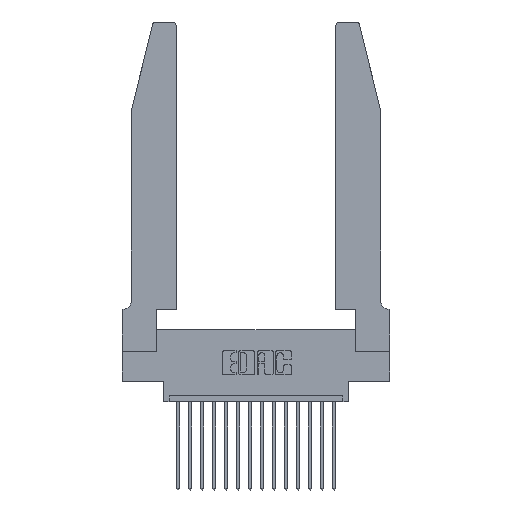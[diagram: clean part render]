
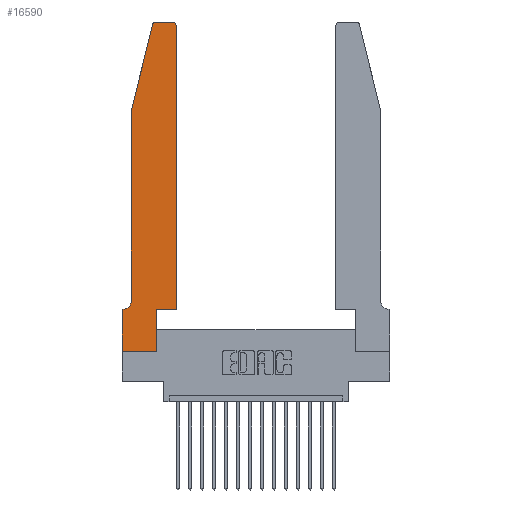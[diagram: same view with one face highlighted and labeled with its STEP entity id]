
A CAD part, top view. The second image highlights one B-rep face of the part: STEP entity #16590.
In plain terms, the highlighted planar face has unit normal (0, 0, 1).
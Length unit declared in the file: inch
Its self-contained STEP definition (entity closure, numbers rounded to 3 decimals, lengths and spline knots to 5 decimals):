
#68 = VECTOR ( 'NONE', #17505, 39.37008 ) ;
#224 = DIRECTION ( 'NONE',  ( 0., -1., 0. ) ) ;
#610 = PLANE ( 'NONE',  #15194 ) ;
#698 = DIRECTION ( 'NONE',  ( 0., 0., 1. ) ) ;
#787 = VECTOR ( 'NONE', #2615, 39.37008 ) ;
#1121 = AXIS2_PLACEMENT_3D ( 'NONE', #5935, #7347, #19142 ) ;
#1133 = CARTESIAN_POINT ( 'NONE',  ( 0.4505, 0.35, 0.37 ) ) ;
#1285 = ORIENTED_EDGE ( 'NONE', *, *, #9515, .T. ) ;
#1320 = CARTESIAN_POINT ( 'NONE',  ( 0.0755, 0.35, 0.37 ) ) ;
#1487 = VERTEX_POINT ( 'NONE', #7179 ) ;
#1521 = CARTESIAN_POINT ( 'NONE',  ( 0., 0., 0.37 ) ) ;
#2225 = ORIENTED_EDGE ( 'NONE', *, *, #17677, .T. ) ;
#2226 = VECTOR ( 'NONE', #9629, 39.37008 ) ;
#2336 = CARTESIAN_POINT ( 'NONE',  ( 0., 0.35, 0.37 ) ) ;
#2412 = CARTESIAN_POINT ( 'NONE',  ( 0., 0.35, 0.37 ) ) ;
#2576 = VECTOR ( 'NONE', #224, 39.37008 ) ;
#2615 = DIRECTION ( 'NONE',  ( 1., 0., 0. ) ) ;
#2790 = DIRECTION ( 'NONE',  ( -1., 0., 0. ) ) ;
#3133 = CARTESIAN_POINT ( 'NONE',  ( 0.0055, 0.42, 0.37 ) ) ;
#3351 = ORIENTED_EDGE ( 'NONE', *, *, #15114, .T. ) ;
#5148 = CARTESIAN_POINT ( 'NONE',  ( 0.2865, 0.35, 0.37 ) ) ;
#5468 = ORIENTED_EDGE ( 'NONE', *, *, #6508, .T. ) ;
#5933 = ORIENTED_EDGE ( 'NONE', *, *, #13284, .T. ) ;
#5935 = CARTESIAN_POINT ( 'NONE',  ( 0.4205, 2.72, 0.37 ) ) ;
#5976 = EDGE_CURVE ( 'NONE', #9731, #7419, #13510, .T. ) ;
#6169 = LINE ( 'NONE', #8352, #2226 ) ;
#6340 = VECTOR ( 'NONE', #11230, 39.37008 ) ;
#6357 = LINE ( 'NONE', #11510, #68 ) ;
#6508 = EDGE_CURVE ( 'NONE', #1487, #10511, #17417, .T. ) ;
#6664 = CARTESIAN_POINT ( 'NONE',  ( 0.284, 2.72, 0.37 ) ) ;
#7179 = CARTESIAN_POINT ( 'NONE',  ( 0.0755, 2., 0.37 ) ) ;
#7347 = DIRECTION ( 'NONE',  ( 0., 0., 1. ) ) ;
#7419 = VERTEX_POINT ( 'NONE', #2336 ) ;
#7518 = DIRECTION ( 'NONE',  ( -1., 0., 0. ) ) ;
#7578 = CARTESIAN_POINT ( 'NONE',  ( 0.0055, 0.35, 0.37 ) ) ;
#8215 = DIRECTION ( 'NONE',  ( 1., 0., 0. ) ) ;
#8330 = CARTESIAN_POINT ( 'NONE',  ( 0.0755, 2., 0.37 ) ) ;
#8352 = CARTESIAN_POINT ( 'NONE',  ( 0.2605, 2.75, 0.37 ) ) ;
#8431 = LINE ( 'NONE', #1133, #787 ) ;
#8439 = ORIENTED_EDGE ( 'NONE', *, *, #9677, .T. ) ;
#8668 = CARTESIAN_POINT ( 'NONE',  ( 0.2865, 0., 0.37 ) ) ;
#8961 = CARTESIAN_POINT ( 'NONE',  ( 0.0755, 2., 0.37 ) ) ;
#9515 = EDGE_CURVE ( 'NONE', #16368, #12347, #6169, .T. ) ;
#9567 = CARTESIAN_POINT ( 'NONE',  ( 0.2865, 0.35, 0.37 ) ) ;
#9583 = VERTEX_POINT ( 'NONE', #8668 ) ;
#9629 = DIRECTION ( 'NONE',  ( -1., 0., 0. ) ) ;
#9677 = EDGE_CURVE ( 'NONE', #10511, #9731, #18678, .T. ) ;
#9731 = VERTEX_POINT ( 'NONE', #7578 ) ;
#9908 = CARTESIAN_POINT ( 'NONE',  ( 0.4505, 0.35, 0.37 ) ) ;
#9911 = AXIS2_PLACEMENT_3D ( 'NONE', #6664, #698, #8215 ) ;
#9961 = DIRECTION ( 'NONE',  ( 1., 0., 0. ) ) ;
#10202 = CARTESIAN_POINT ( 'NONE',  ( 0.4505, 0.35, 0.37 ) ) ;
#10223 = VECTOR ( 'NONE', #19136, 39.37008 ) ;
#10240 = LINE ( 'NONE', #8330, #6340 ) ;
#10306 = CIRCLE ( 'NONE', #9911, 0.03 ) ;
#10511 = VERTEX_POINT ( 'NONE', #10960 ) ;
#10517 = ORIENTED_EDGE ( 'NONE', *, *, #5976, .T. ) ;
#10960 = CARTESIAN_POINT ( 'NONE',  ( 0.0755, 0.42, 0.37 ) ) ;
#11083 = EDGE_LOOP ( 'NONE', ( #1285, #14892, #14658, #5468, #8439, #10517, #15451, #3351, #18061, #2225, #18205, #5933 ) ) ;
#11178 = LINE ( 'NONE', #10202, #13794 ) ;
#11230 = DIRECTION ( 'NONE',  ( -0.239, -0.971, 0. ) ) ;
#11510 = CARTESIAN_POINT ( 'NONE',  ( 0., 0., 0.37 ) ) ;
#11709 = DIRECTION ( 'NONE',  ( 0., 1., 0. ) ) ;
#12335 = EDGE_CURVE ( 'NONE', #12347, #12551, #10306, .T. ) ;
#12347 = VERTEX_POINT ( 'NONE', #17155 ) ;
#12449 = CARTESIAN_POINT ( 'NONE',  ( 0.4505, 2.72, 0.37 ) ) ;
#12551 = VERTEX_POINT ( 'NONE', #14620 ) ;
#12787 = VECTOR ( 'NONE', #2790, 39.37008 ) ;
#13284 = EDGE_CURVE ( 'NONE', #18165, #16368, #17490, .T. ) ;
#13477 = EDGE_CURVE ( 'NONE', #9583, #13559, #18426, .T. ) ;
#13495 = DIRECTION ( 'NONE',  ( 0., 0., -1. ) ) ;
#13510 = LINE ( 'NONE', #1320, #12787 ) ;
#13559 = VERTEX_POINT ( 'NONE', #5148 ) ;
#13794 = VECTOR ( 'NONE', #11709, 39.37008 ) ;
#13815 = EDGE_CURVE ( 'NONE', #7419, #14079, #6357, .T. ) ;
#13839 = EDGE_CURVE ( 'NONE', #17670, #18165, #11178, .T. ) ;
#14026 = VECTOR ( 'NONE', #18356, 39.37008 ) ;
#14079 = VERTEX_POINT ( 'NONE', #14124 ) ;
#14124 = CARTESIAN_POINT ( 'NONE',  ( 0., 0., 0.37 ) ) ;
#14207 = LINE ( 'NONE', #1521, #10223 ) ;
#14620 = CARTESIAN_POINT ( 'NONE',  ( 0.25487, 2.72718, 0.37 ) ) ;
#14658 = ORIENTED_EDGE ( 'NONE', *, *, #18542, .T. ) ;
#14892 = ORIENTED_EDGE ( 'NONE', *, *, #12335, .T. ) ;
#15114 = EDGE_CURVE ( 'NONE', #14079, #9583, #14207, .T. ) ;
#15194 = AXIS2_PLACEMENT_3D ( 'NONE', #2412, #17188, #9961 ) ;
#15451 = ORIENTED_EDGE ( 'NONE', *, *, #13815, .T. ) ;
#16294 = AXIS2_PLACEMENT_3D ( 'NONE', #3133, #13495, #7518 ) ;
#16368 = VERTEX_POINT ( 'NONE', #18005 ) ;
#16590 = ADVANCED_FACE ( 'NONE', ( #16700 ), #610, .T. ) ;
#16700 = FACE_OUTER_BOUND ( 'NONE', #11083, .T. ) ;
#17155 = CARTESIAN_POINT ( 'NONE',  ( 0.284, 2.75, 0.37 ) ) ;
#17188 = DIRECTION ( 'NONE',  ( 0., 0., 1. ) ) ;
#17417 = LINE ( 'NONE', #8961, #2576 ) ;
#17490 = CIRCLE ( 'NONE', #1121, 0.03 ) ;
#17505 = DIRECTION ( 'NONE',  ( 0., -1., 0. ) ) ;
#17670 = VERTEX_POINT ( 'NONE', #9908 ) ;
#17677 = EDGE_CURVE ( 'NONE', #13559, #17670, #8431, .T. ) ;
#18005 = CARTESIAN_POINT ( 'NONE',  ( 0.4205, 2.75, 0.37 ) ) ;
#18061 = ORIENTED_EDGE ( 'NONE', *, *, #13477, .T. ) ;
#18165 = VERTEX_POINT ( 'NONE', #12449 ) ;
#18205 = ORIENTED_EDGE ( 'NONE', *, *, #13839, .T. ) ;
#18356 = DIRECTION ( 'NONE',  ( 0., 1., 0. ) ) ;
#18426 = LINE ( 'NONE', #9567, #14026 ) ;
#18542 = EDGE_CURVE ( 'NONE', #12551, #1487, #10240, .T. ) ;
#18678 = CIRCLE ( 'NONE', #16294, 0.07 ) ;
#19136 = DIRECTION ( 'NONE',  ( 1., 0., 0. ) ) ;
#19142 = DIRECTION ( 'NONE',  ( 1., 0., 0. ) ) ;
